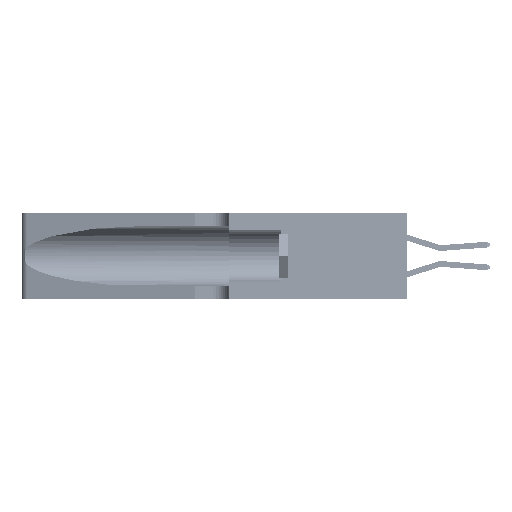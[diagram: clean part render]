
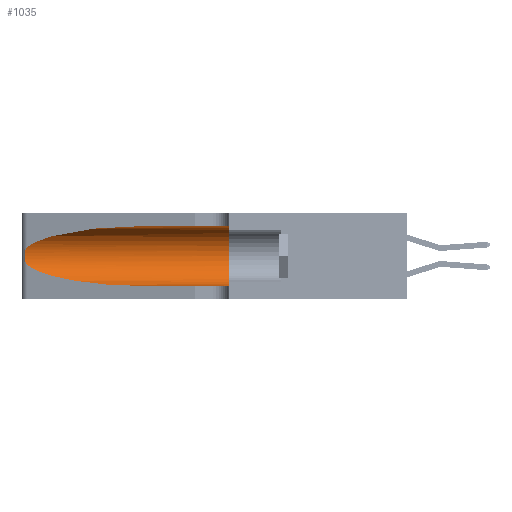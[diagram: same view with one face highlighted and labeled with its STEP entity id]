
A CAD part, left-side view. The second image highlights one B-rep face of the part: STEP entity #1035.
In plain terms, the highlighted cylindrical face has radius 3.308 mm (diameter 6.617 mm), a partial arc.
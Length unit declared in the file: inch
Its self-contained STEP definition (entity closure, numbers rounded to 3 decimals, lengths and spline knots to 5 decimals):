
#1035 = ADVANCED_FACE ( 'NONE', ( #27483 ), #8993, .F. ) ;
#2741 = CARTESIAN_POINT ( 'NONE',  ( 0.25856, 1.23593, 0.16098 ) ) ;
#2818 = ORIENTED_EDGE ( 'NONE', *, *, #15752, .F. ) ;
#2859 = CARTESIAN_POINT ( 'NONE',  ( 0.25487, 1.22718, 0.14631 ) ) ;
#3073 = CARTESIAN_POINT ( 'NONE',  ( 0.25487, 1.22718, 0.14631 ) ) ;
#6305 =( BOUNDED_CURVE ( )  B_SPLINE_CURVE ( 3, ( #2859, #22622, #15018, #34487 ),
 .UNSPECIFIED., .F., .T. ) 
 B_SPLINE_CURVE_WITH_KNOTS ( ( 4, 4 ),
 ( 3.44316, 4.71239 ),
 .UNSPECIFIED. ) 
 CURVE ( )  GEOMETRIC_REPRESENTATION_ITEM ( )  RATIONAL_B_SPLINE_CURVE ( ( 1., 0.87, 0.87, 1. ) ) 
 REPRESENTATION_ITEM ( '' )  );
#6912 = CARTESIAN_POINT ( 'NONE',  ( 0.1305, 0.72297, 0.31525 ) ) ;
#7037 = CARTESIAN_POINT ( 'NONE',  ( 0.1305, 0.72297, 0.05475 ) ) ;
#7062 = ORIENTED_EDGE ( 'NONE', *, *, #11682, .T. ) ;
#7865 = CARTESIAN_POINT ( 'NONE',  ( 0.18966, 0.96281, 0.31525 ) ) ;
#8810 = VERTEX_POINT ( 'NONE', #19132 ) ;
#8993 = CYLINDRICAL_SURFACE ( 'NONE', #16074, 0.13025 ) ;
#9806 = CARTESIAN_POINT ( 'NONE',  ( 0.1305, 1.61858, 0.185 ) ) ;
#10726 = EDGE_CURVE ( 'NONE', #39316, #14489, #6305, .T. ) ;
#10949 = CARTESIAN_POINT ( 'NONE',  ( 0.25639, 1.23184, 0.21858 ) ) ;
#11682 = EDGE_CURVE ( 'NONE', #14489, #50275, #17890, .T. ) ;
#12338 = CARTESIAN_POINT ( 'NONE',  ( 0.1305, 1.61858, 0.05475 ) ) ;
#13877 =( BOUNDED_CURVE ( )  B_SPLINE_CURVE ( 3, ( #47130, #7865, #47463, #36262 ),
 .UNSPECIFIED., .F., .F. ) 
 B_SPLINE_CURVE_WITH_KNOTS ( ( 4, 4 ),
 ( 1.5708, 2.84003 ),
 .UNSPECIFIED. ) 
 CURVE ( )  GEOMETRIC_REPRESENTATION_ITEM ( )  RATIONAL_B_SPLINE_CURVE ( ( 1., 0.87, 0.87, 1. ) ) 
 REPRESENTATION_ITEM ( '' )  );
#13921 = ORIENTED_EDGE ( 'NONE', *, *, #10726, .T. ) ;
#14291 = VERTEX_POINT ( 'NONE', #31999 ) ;
#14489 = VERTEX_POINT ( 'NONE', #7037 ) ;
#14571 = CARTESIAN_POINT ( 'NONE',  ( 0.25787, 1.23484, 0.2124 ) ) ;
#14735 = CARTESIAN_POINT ( 'NONE',  ( 0.26075, 1.23896, 0.19203 ) ) ;
#14896 = CARTESIAN_POINT ( 'NONE',  ( 0.26075, 1.23896, 0.178 ) ) ;
#15018 = CARTESIAN_POINT ( 'NONE',  ( 0.18966, 0.96281, 0.05475 ) ) ;
#15752 = EDGE_CURVE ( 'NONE', #28502, #14291, #23619, .T. ) ;
#16074 = AXIS2_PLACEMENT_3D ( 'NONE', #9806, #41302, #17729 ) ;
#17402 = CARTESIAN_POINT ( 'NONE',  ( 0.1305, 0.35, 0.185 ) ) ;
#17729 = DIRECTION ( 'NONE',  ( 0., 0., -1. ) ) ;
#17890 = LINE ( 'NONE', #12338, #24654 ) ;
#19132 = CARTESIAN_POINT ( 'NONE',  ( 0.25487, 1.22718, 0.22369 ) ) ;
#19900 = VECTOR ( 'NONE', #29154, 39.37008 ) ;
#22512 = CARTESIAN_POINT ( 'NONE',  ( 0.25854, 1.2359, 0.20912 ) ) ;
#22622 = CARTESIAN_POINT ( 'NONE',  ( 0.2373, 1.15595, 0.08982 ) ) ;
#23619 = LINE ( 'NONE', #25014, #19900 ) ;
#24654 = VECTOR ( 'NONE', #48006, 39.37008 ) ;
#25014 = CARTESIAN_POINT ( 'NONE',  ( 0.1305, 1.61858, 0.31525 ) ) ;
#25470 = ORIENTED_EDGE ( 'NONE', *, *, #43632, .F. ) ;
#25577 = AXIS2_PLACEMENT_3D ( 'NONE', #17402, #48937, #37046 ) ;
#26627 = CARTESIAN_POINT ( 'NONE',  ( 0.25789, 1.23486, 0.15765 ) ) ;
#27483 = FACE_OUTER_BOUND ( 'NONE', #43254, .T. ) ;
#28502 = VERTEX_POINT ( 'NONE', #6912 ) ;
#29154 = DIRECTION ( 'NONE',  ( 0., -1., 0. ) ) ;
#29508 = CARTESIAN_POINT ( 'NONE',  ( 0.25487, 1.22718, 0.14631 ) ) ;
#31999 = CARTESIAN_POINT ( 'NONE',  ( 0.1305, 0.35, 0.31525 ) ) ;
#34215 = CARTESIAN_POINT ( 'NONE',  ( 0.26018, 1.23835, 0.19895 ) ) ;
#34408 = B_SPLINE_CURVE_WITH_KNOTS ( 'NONE', 3,
 ( #34863, #38347, #10949, #14571, #22512, #34215, #14735, #14896, #50233, #2741, #26627, #38512, #45905, #3073 ),
 .UNSPECIFIED., .F., .F.,
 ( 4, 2, 2, 2, 2, 2, 4 ),
 ( 0., 0.00027, 0.00053, 0.00107, 0.0016, 0.00187, 0.00214 ),
 .UNSPECIFIED. ) ;
#34487 = CARTESIAN_POINT ( 'NONE',  ( 0.1305, 0.72297, 0.05475 ) ) ;
#34863 = CARTESIAN_POINT ( 'NONE',  ( 0.25487, 1.22718, 0.22369 ) ) ;
#36262 = CARTESIAN_POINT ( 'NONE',  ( 0.25487, 1.22718, 0.22369 ) ) ;
#37046 = DIRECTION ( 'NONE',  ( 0., 0., 1. ) ) ;
#38347 = CARTESIAN_POINT ( 'NONE',  ( 0.25555, 1.22994, 0.2215 ) ) ;
#38512 = CARTESIAN_POINT ( 'NONE',  ( 0.25639, 1.23186, 0.15144 ) ) ;
#39316 = VERTEX_POINT ( 'NONE', #29508 ) ;
#39886 = EDGE_CURVE ( 'NONE', #28502, #8810, #13877, .T. ) ;
#40239 = EDGE_CURVE ( 'NONE', #8810, #39316, #34408, .T. ) ;
#41302 = DIRECTION ( 'NONE',  ( 0., -1., 0. ) ) ;
#41980 = ORIENTED_EDGE ( 'NONE', *, *, #40239, .T. ) ;
#43254 = EDGE_LOOP ( 'NONE', ( #44760, #41980, #13921, #7062, #25470, #2818 ) ) ;
#43347 = CARTESIAN_POINT ( 'NONE',  ( 0.1305, 0.35, 0.05475 ) ) ;
#43632 = EDGE_CURVE ( 'NONE', #14291, #50275, #44556, .T. ) ;
#44556 = CIRCLE ( 'NONE', #25577, 0.13025 ) ;
#44760 = ORIENTED_EDGE ( 'NONE', *, *, #39886, .T. ) ;
#45905 = CARTESIAN_POINT ( 'NONE',  ( 0.25555, 1.22993, 0.14849 ) ) ;
#47130 = CARTESIAN_POINT ( 'NONE',  ( 0.1305, 0.72297, 0.31525 ) ) ;
#47463 = CARTESIAN_POINT ( 'NONE',  ( 0.2373, 1.15595, 0.28018 ) ) ;
#48006 = DIRECTION ( 'NONE',  ( 0., -1., 0. ) ) ;
#48937 = DIRECTION ( 'NONE',  ( 0., 1., 0. ) ) ;
#50233 = CARTESIAN_POINT ( 'NONE',  ( 0.26017, 1.23833, 0.17102 ) ) ;
#50275 = VERTEX_POINT ( 'NONE', #43347 ) ;
